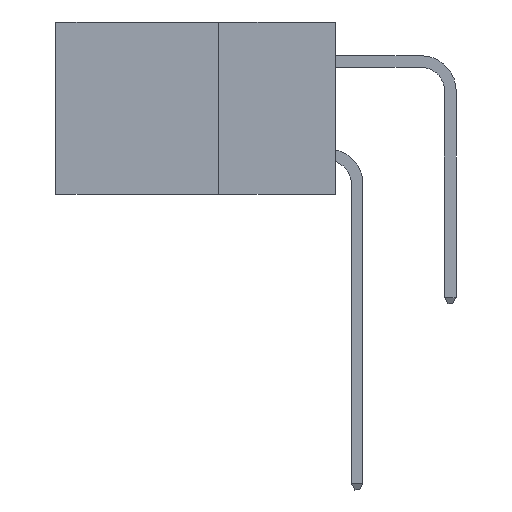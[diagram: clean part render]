
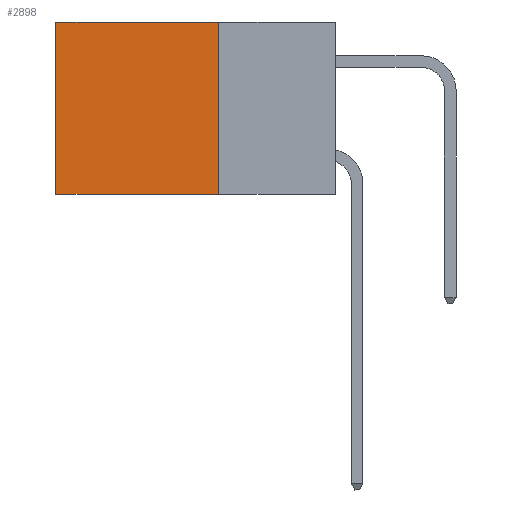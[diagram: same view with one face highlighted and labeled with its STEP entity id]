
A CAD part, left-side view. The second image highlights one B-rep face of the part: STEP entity #2898.
In plain terms, the highlighted planar face has unit normal (-1, 0, 0).
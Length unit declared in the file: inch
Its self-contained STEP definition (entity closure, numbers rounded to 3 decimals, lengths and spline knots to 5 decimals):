
#272 = LINE ( 'NONE', #8897, #1865 ) ;
#635 = VERTEX_POINT ( 'NONE', #17989 ) ;
#1865 = VECTOR ( 'NONE', #2565, 39.37008 ) ;
#1918 = ORIENTED_EDGE ( 'NONE', *, *, #25491, .F. ) ;
#2565 = DIRECTION ( 'NONE',  ( 0., 0., -1. ) ) ;
#2898 = ADVANCED_FACE ( 'NONE', ( #10160 ), #9871, .F. ) ;
#3866 = EDGE_CURVE ( 'NONE', #635, #17027, #21979, .T. ) ;
#4077 = EDGE_CURVE ( 'NONE', #635, #21150, #24643, .T. ) ;
#7429 = VERTEX_POINT ( 'NONE', #19237 ) ;
#8046 = DIRECTION ( 'NONE',  ( 0., 0., -1. ) ) ;
#8897 = CARTESIAN_POINT ( 'NONE',  ( 0.2875, 0.6, 0. ) ) ;
#9283 = CARTESIAN_POINT ( 'NONE',  ( 0.2875, 0.25, 0. ) ) ;
#9420 = DIRECTION ( 'NONE',  ( 0., 0., -1. ) ) ;
#9871 = PLANE ( 'NONE',  #20461 ) ;
#10160 = FACE_OUTER_BOUND ( 'NONE', #21556, .T. ) ;
#11558 = DIRECTION ( 'NONE',  ( 0., 1., 0. ) ) ;
#13665 = CARTESIAN_POINT ( 'NONE',  ( 0.2875, 0.25, -0.37 ) ) ;
#13892 = ORIENTED_EDGE ( 'NONE', *, *, #16499, .T. ) ;
#14085 = ORIENTED_EDGE ( 'NONE', *, *, #4077, .F. ) ;
#14692 = DIRECTION ( 'NONE',  ( 1., 0., 0. ) ) ;
#14944 = VECTOR ( 'NONE', #9420, 39.37008 ) ;
#15475 = ORIENTED_EDGE ( 'NONE', *, *, #3866, .T. ) ;
#16499 = EDGE_CURVE ( 'NONE', #17027, #7429, #272, .T. ) ;
#17027 = VERTEX_POINT ( 'NONE', #17473 ) ;
#17029 = VECTOR ( 'NONE', #11558, 39.37008 ) ;
#17473 = CARTESIAN_POINT ( 'NONE',  ( 0.2875, 0.6, 0. ) ) ;
#17580 = DIRECTION ( 'NONE',  ( 0., 1., 0. ) ) ;
#17989 = CARTESIAN_POINT ( 'NONE',  ( 0.2875, 0.25, 0. ) ) ;
#18146 = CARTESIAN_POINT ( 'NONE',  ( 0.2875, 0.25, 0. ) ) ;
#18496 = VECTOR ( 'NONE', #17580, 39.37008 ) ;
#19237 = CARTESIAN_POINT ( 'NONE',  ( 0.2875, 0.6, -0.37 ) ) ;
#20461 = AXIS2_PLACEMENT_3D ( 'NONE', #23279, #14692, #8046 ) ;
#21150 = VERTEX_POINT ( 'NONE', #22936 ) ;
#21556 = EDGE_LOOP ( 'NONE', ( #13892, #1918, #14085, #15475 ) ) ;
#21979 = LINE ( 'NONE', #9283, #18496 ) ;
#22936 = CARTESIAN_POINT ( 'NONE',  ( 0.2875, 0.25, -0.37 ) ) ;
#23279 = CARTESIAN_POINT ( 'NONE',  ( 0.2875, 0.25, 0. ) ) ;
#24524 = LINE ( 'NONE', #13665, #17029 ) ;
#24643 = LINE ( 'NONE', #18146, #14944 ) ;
#25491 = EDGE_CURVE ( 'NONE', #21150, #7429, #24524, .T. ) ;
